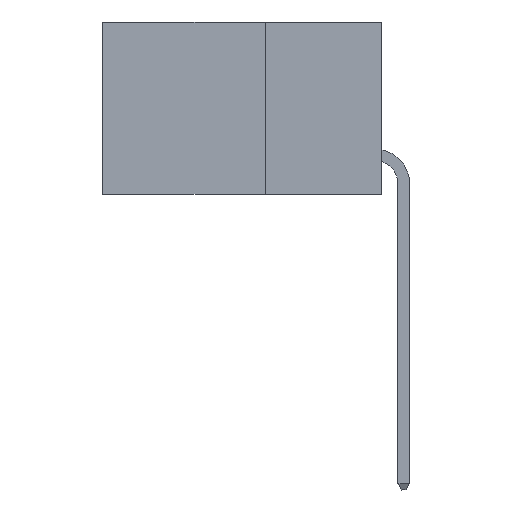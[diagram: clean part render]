
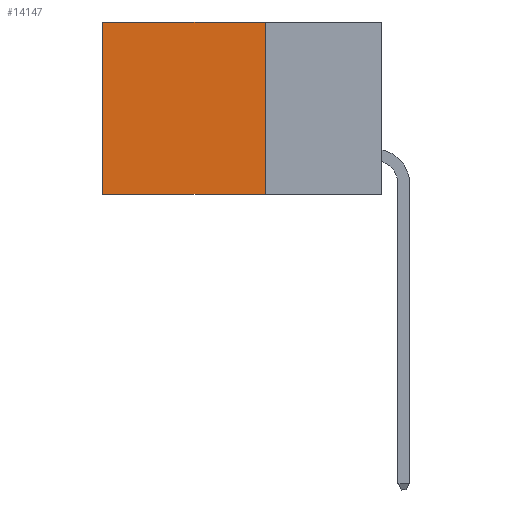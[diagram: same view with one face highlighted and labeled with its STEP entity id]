
A CAD part, left-side view. The second image highlights one B-rep face of the part: STEP entity #14147.
In plain terms, the highlighted planar face has unit normal (-1, 0, 0).
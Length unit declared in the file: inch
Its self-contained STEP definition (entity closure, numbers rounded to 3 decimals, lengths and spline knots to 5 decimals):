
#724 = ORIENTED_EDGE ( 'NONE', *, *, #27207, .F. ) ;
#1474 = LINE ( 'NONE', #25810, #12422 ) ;
#2853 = LINE ( 'NONE', #27574, #25085 ) ;
#3327 = VERTEX_POINT ( 'NONE', #15511 ) ;
#3542 = DIRECTION ( 'NONE',  ( 0., 0., -1. ) ) ;
#4226 = EDGE_CURVE ( 'NONE', #21165, #17328, #2853, .T. ) ;
#5149 = LINE ( 'NONE', #5742, #16031 ) ;
#5324 = PLANE ( 'NONE',  #22391 ) ;
#5742 = CARTESIAN_POINT ( 'NONE',  ( 0.2875, 0.6, 0. ) ) ;
#7562 = CARTESIAN_POINT ( 'NONE',  ( 0.2875, 0.25, 0. ) ) ;
#8341 = ORIENTED_EDGE ( 'NONE', *, *, #21291, .T. ) ;
#9823 = FACE_OUTER_BOUND ( 'NONE', #25343, .T. ) ;
#11929 = DIRECTION ( 'NONE',  ( 1., 0., 0. ) ) ;
#12422 = VECTOR ( 'NONE', #25494, 39.37008 ) ;
#12535 = VERTEX_POINT ( 'NONE', #21064 ) ;
#12549 = CARTESIAN_POINT ( 'NONE',  ( 0.2875, 0.25, 0. ) ) ;
#12674 = DIRECTION ( 'NONE',  ( 0., 0., -1. ) ) ;
#14040 = ORIENTED_EDGE ( 'NONE', *, *, #4226, .F. ) ;
#14147 = ADVANCED_FACE ( 'NONE', ( #9823 ), #5324, .F. ) ;
#14850 = VECTOR ( 'NONE', #19002, 39.37008 ) ;
#15004 = EDGE_CURVE ( 'NONE', #21165, #3327, #20520, .T. ) ;
#15511 = CARTESIAN_POINT ( 'NONE',  ( 0.2875, 0.6, 0. ) ) ;
#16031 = VECTOR ( 'NONE', #3542, 39.37008 ) ;
#17230 = ORIENTED_EDGE ( 'NONE', *, *, #15004, .T. ) ;
#17328 = VERTEX_POINT ( 'NONE', #27827 ) ;
#18303 = CARTESIAN_POINT ( 'NONE',  ( 0.2875, 0.25, 0. ) ) ;
#19002 = DIRECTION ( 'NONE',  ( 0., 1., 0. ) ) ;
#20520 = LINE ( 'NONE', #12549, #14850 ) ;
#21064 = CARTESIAN_POINT ( 'NONE',  ( 0.2875, 0.6, -0.37 ) ) ;
#21165 = VERTEX_POINT ( 'NONE', #7562 ) ;
#21291 = EDGE_CURVE ( 'NONE', #3327, #12535, #5149, .T. ) ;
#22391 = AXIS2_PLACEMENT_3D ( 'NONE', #18303, #11929, #26824 ) ;
#25085 = VECTOR ( 'NONE', #12674, 39.37008 ) ;
#25343 = EDGE_LOOP ( 'NONE', ( #8341, #724, #14040, #17230 ) ) ;
#25494 = DIRECTION ( 'NONE',  ( 0., 1., 0. ) ) ;
#25810 = CARTESIAN_POINT ( 'NONE',  ( 0.2875, 0.25, -0.37 ) ) ;
#26824 = DIRECTION ( 'NONE',  ( 0., 0., -1. ) ) ;
#27207 = EDGE_CURVE ( 'NONE', #17328, #12535, #1474, .T. ) ;
#27574 = CARTESIAN_POINT ( 'NONE',  ( 0.2875, 0.25, 0. ) ) ;
#27827 = CARTESIAN_POINT ( 'NONE',  ( 0.2875, 0.25, -0.37 ) ) ;
